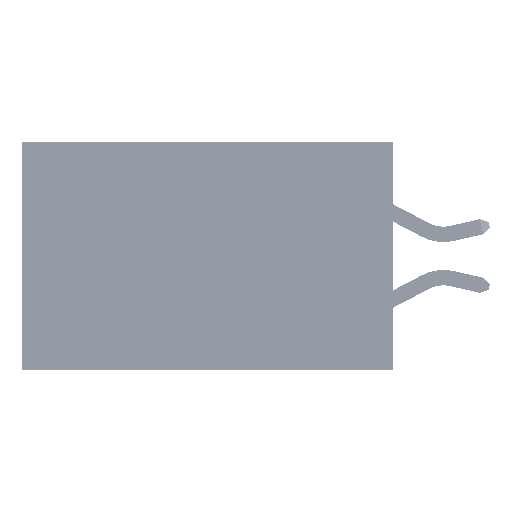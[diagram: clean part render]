
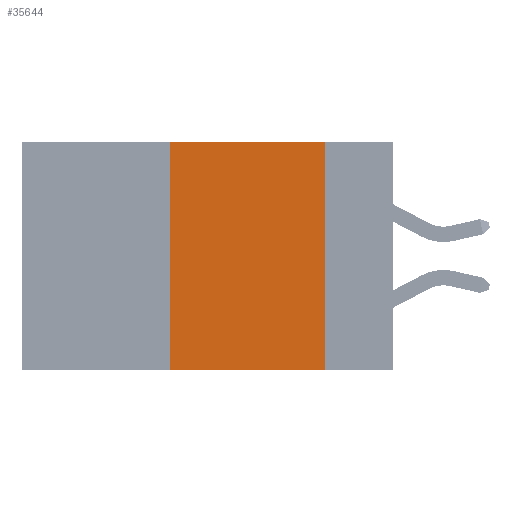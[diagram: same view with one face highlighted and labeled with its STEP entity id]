
A CAD part, left-side view. The second image highlights one B-rep face of the part: STEP entity #35644.
In plain terms, the highlighted planar face has unit normal (-1, 0, 0).
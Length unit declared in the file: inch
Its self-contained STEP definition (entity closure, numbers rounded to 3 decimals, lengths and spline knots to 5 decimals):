
#1313 = ORIENTED_EDGE ( 'NONE', *, *, #21116, .F. ) ;
#2244 = EDGE_CURVE ( 'NONE', #5440, #22553, #40017, .T. ) ;
#5128 = VERTEX_POINT ( 'NONE', #5207 ) ;
#5207 = CARTESIAN_POINT ( 'NONE',  ( 0., 0.11, 0. ) ) ;
#5440 = VERTEX_POINT ( 'NONE', #37248 ) ;
#6063 = FACE_OUTER_BOUND ( 'NONE', #20609, .T. ) ;
#7266 = VECTOR ( 'NONE', #39896, 39.37008 ) ;
#8231 = DIRECTION ( 'NONE',  ( 0., 0., 1. ) ) ;
#8730 = EDGE_CURVE ( 'NONE', #40424, #5128, #35469, .T. ) ;
#9653 = PLANE ( 'NONE',  #22087 ) ;
#13295 = VECTOR ( 'NONE', #33261, 39.37008 ) ;
#15481 = CARTESIAN_POINT ( 'NONE',  ( 0., 0.11, -0.37 ) ) ;
#15876 = DIRECTION ( 'NONE',  ( 1., 0., 0. ) ) ;
#19298 = EDGE_CURVE ( 'NONE', #5128, #22553, #38767, .T. ) ;
#19444 = CARTESIAN_POINT ( 'NONE',  ( 0., 0.6, 0. ) ) ;
#19941 = CARTESIAN_POINT ( 'NONE',  ( 0., 0.6, 0. ) ) ;
#20120 = CARTESIAN_POINT ( 'NONE',  ( 0., 0.6, -0.37 ) ) ;
#20609 = EDGE_LOOP ( 'NONE', ( #21540, #38858, #1313, #20818 ) ) ;
#20818 = ORIENTED_EDGE ( 'NONE', *, *, #2244, .T. ) ;
#21116 = EDGE_CURVE ( 'NONE', #5440, #40424, #35766, .T. ) ;
#21540 = ORIENTED_EDGE ( 'NONE', *, *, #19298, .F. ) ;
#22087 = AXIS2_PLACEMENT_3D ( 'NONE', #19444, #15876, #43156 ) ;
#22553 = VERTEX_POINT ( 'NONE', #15481 ) ;
#27856 = CARTESIAN_POINT ( 'NONE',  ( 0., 0.36, 0. ) ) ;
#30366 = DIRECTION ( 'NONE',  ( 0., 0., -1. ) ) ;
#33261 = DIRECTION ( 'NONE',  ( 0., -1., 0. ) ) ;
#34715 = VECTOR ( 'NONE', #8231, 39.37008 ) ;
#35469 = LINE ( 'NONE', #19941, #13295 ) ;
#35644 = ADVANCED_FACE ( 'NONE', ( #6063 ), #9653, .F. ) ;
#35766 = LINE ( 'NONE', #38374, #34715 ) ;
#36182 = VECTOR ( 'NONE', #30366, 39.37008 ) ;
#37152 = CARTESIAN_POINT ( 'NONE',  ( 0., 0.11, 0. ) ) ;
#37248 = CARTESIAN_POINT ( 'NONE',  ( 0., 0.36, -0.37 ) ) ;
#38374 = CARTESIAN_POINT ( 'NONE',  ( 0., 0.36, 0. ) ) ;
#38767 = LINE ( 'NONE', #37152, #36182 ) ;
#38858 = ORIENTED_EDGE ( 'NONE', *, *, #8730, .F. ) ;
#39896 = DIRECTION ( 'NONE',  ( 0., -1., 0. ) ) ;
#40017 = LINE ( 'NONE', #20120, #7266 ) ;
#40424 = VERTEX_POINT ( 'NONE', #27856 ) ;
#43156 = DIRECTION ( 'NONE',  ( 0., 0., -1. ) ) ;
